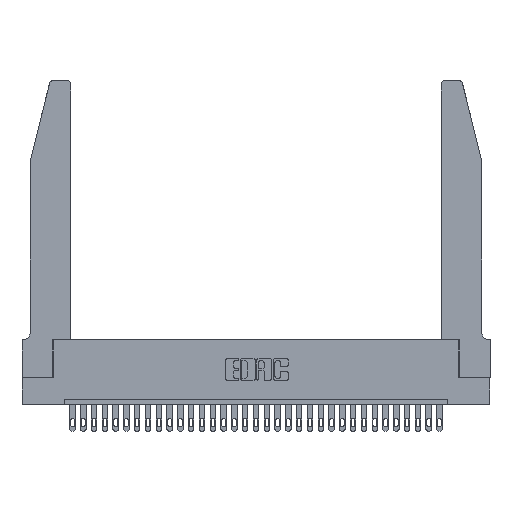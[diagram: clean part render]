
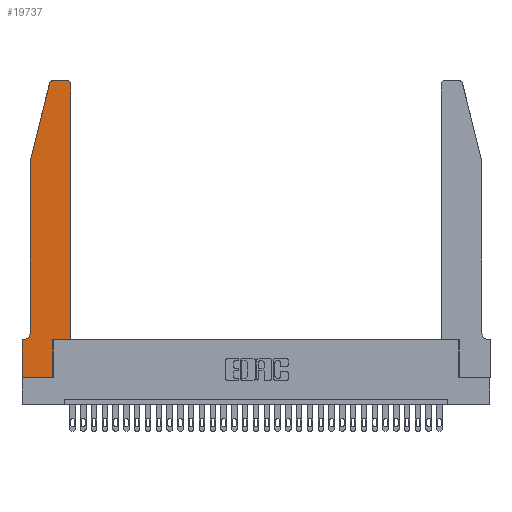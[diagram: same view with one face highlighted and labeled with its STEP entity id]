
A CAD part, top view. The second image highlights one B-rep face of the part: STEP entity #19737.
In plain terms, the highlighted planar face has unit normal (0, 0, 1).
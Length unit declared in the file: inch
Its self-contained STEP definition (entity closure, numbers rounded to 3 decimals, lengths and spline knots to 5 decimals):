
#480 = CARTESIAN_POINT ( 'NONE',  ( 0.0755, 2., 0.37 ) ) ;
#620 = CARTESIAN_POINT ( 'NONE',  ( 0.2605, 2.75, 0.37 ) ) ;
#702 = DIRECTION ( 'NONE',  ( -1., 0., 0. ) ) ;
#852 = CARTESIAN_POINT ( 'NONE',  ( 0., 0.35, 0.37 ) ) ;
#1043 = CARTESIAN_POINT ( 'NONE',  ( 0.0755, 0.42, 0.37 ) ) ;
#1354 = EDGE_CURVE ( 'NONE', #4685, #29435, #10092, .T. ) ;
#1769 = VERTEX_POINT ( 'NONE', #21962 ) ;
#2161 = EDGE_CURVE ( 'NONE', #25814, #4685, #17401, .T. ) ;
#2684 = VERTEX_POINT ( 'NONE', #5732 ) ;
#3289 = DIRECTION ( 'NONE',  ( 0., -1., 0. ) ) ;
#3474 = ORIENTED_EDGE ( 'NONE', *, *, #5643, .T. ) ;
#3964 = LINE ( 'NONE', #4809, #13573 ) ;
#4007 = CARTESIAN_POINT ( 'NONE',  ( 0.4505, 0.35, 0.37 ) ) ;
#4215 = ORIENTED_EDGE ( 'NONE', *, *, #8852, .T. ) ;
#4258 = ORIENTED_EDGE ( 'NONE', *, *, #21538, .T. ) ;
#4620 = EDGE_CURVE ( 'NONE', #2684, #25814, #16845, .T. ) ;
#4685 = VERTEX_POINT ( 'NONE', #16124 ) ;
#4809 = CARTESIAN_POINT ( 'NONE',  ( 0.4505, 0.35, 0.37 ) ) ;
#4876 = ORIENTED_EDGE ( 'NONE', *, *, #26256, .T. ) ;
#4889 = ORIENTED_EDGE ( 'NONE', *, *, #4620, .T. ) ;
#5631 = CARTESIAN_POINT ( 'NONE',  ( 0., 0.35, 0.37 ) ) ;
#5643 = EDGE_CURVE ( 'NONE', #20206, #14360, #23951, .T. ) ;
#5732 = CARTESIAN_POINT ( 'NONE',  ( 0., 0., 0.37 ) ) ;
#5796 = CARTESIAN_POINT ( 'NONE',  ( 0.0055, 0.42, 0.37 ) ) ;
#6138 = VECTOR ( 'NONE', #3289, 39.37008 ) ;
#7072 = AXIS2_PLACEMENT_3D ( 'NONE', #5796, #15475, #702 ) ;
#8675 = VERTEX_POINT ( 'NONE', #22798 ) ;
#8722 = EDGE_CURVE ( 'NONE', #1769, #20276, #18851, .T. ) ;
#8852 = EDGE_CURVE ( 'NONE', #15446, #24957, #28484, .T. ) ;
#8930 = DIRECTION ( 'NONE',  ( 0., 1., 0. ) ) ;
#9230 = DIRECTION ( 'NONE',  ( -0.239, -0.971, 0. ) ) ;
#10092 = LINE ( 'NONE', #4007, #18231 ) ;
#10106 = ORIENTED_EDGE ( 'NONE', *, *, #26439, .T. ) ;
#10431 = LINE ( 'NONE', #620, #18953 ) ;
#11023 = DIRECTION ( 'NONE',  ( 1., 0., 0. ) ) ;
#11330 = CIRCLE ( 'NONE', #7072, 0.07 ) ;
#11789 = CARTESIAN_POINT ( 'NONE',  ( 0.2865, 0., 0.37 ) ) ;
#11994 = DIRECTION ( 'NONE',  ( 1., 0., 0. ) ) ;
#12185 = ORIENTED_EDGE ( 'NONE', *, *, #26866, .T. ) ;
#12751 = FACE_OUTER_BOUND ( 'NONE', #15650, .T. ) ;
#13332 = CARTESIAN_POINT ( 'NONE',  ( 0.284, 2.72, 0.37 ) ) ;
#13545 = EDGE_CURVE ( 'NONE', #24957, #8675, #10431, .T. ) ;
#13573 = VECTOR ( 'NONE', #22075, 39.37008 ) ;
#13743 = CARTESIAN_POINT ( 'NONE',  ( 0.2865, 0.35, 0.37 ) ) ;
#14101 = VERTEX_POINT ( 'NONE', #1043 ) ;
#14218 = CARTESIAN_POINT ( 'NONE',  ( 0.4505, 2.72, 0.37 ) ) ;
#14225 = LINE ( 'NONE', #15565, #6138 ) ;
#14360 = VERTEX_POINT ( 'NONE', #480 ) ;
#15446 = VERTEX_POINT ( 'NONE', #14218 ) ;
#15475 = DIRECTION ( 'NONE',  ( 0., 0., -1. ) ) ;
#15504 = CIRCLE ( 'NONE', #27326, 0.03 ) ;
#15565 = CARTESIAN_POINT ( 'NONE',  ( 0., 0., 0.37 ) ) ;
#15650 = EDGE_LOOP ( 'NONE', ( #23477, #12185, #3474, #4876, #25760, #18470, #4258, #4889, #22389, #18075, #10106, #4215 ) ) ;
#15756 = CARTESIAN_POINT ( 'NONE',  ( 0.25487, 2.72718, 0.37 ) ) ;
#16124 = CARTESIAN_POINT ( 'NONE',  ( 0.2865, 0.35, 0.37 ) ) ;
#16845 = LINE ( 'NONE', #18393, #20302 ) ;
#16876 = DIRECTION ( 'NONE',  ( 0., 0., 1. ) ) ;
#17401 = LINE ( 'NONE', #13743, #28562 ) ;
#17899 = DIRECTION ( 'NONE',  ( -1., 0., 0. ) ) ;
#18075 = ORIENTED_EDGE ( 'NONE', *, *, #1354, .T. ) ;
#18154 = AXIS2_PLACEMENT_3D ( 'NONE', #852, #23378, #25742 ) ;
#18231 = VECTOR ( 'NONE', #19000, 39.37008 ) ;
#18257 = DIRECTION ( 'NONE',  ( 0., 0., 1. ) ) ;
#18393 = CARTESIAN_POINT ( 'NONE',  ( 0., 0., 0.37 ) ) ;
#18470 = ORIENTED_EDGE ( 'NONE', *, *, #8722, .T. ) ;
#18851 = LINE ( 'NONE', #20424, #28876 ) ;
#18953 = VECTOR ( 'NONE', #17899, 39.37008 ) ;
#19000 = DIRECTION ( 'NONE',  ( 1., 0., 0. ) ) ;
#19737 = ADVANCED_FACE ( 'NONE', ( #12751 ), #27813, .T. ) ;
#20206 = VERTEX_POINT ( 'NONE', #15756 ) ;
#20276 = VERTEX_POINT ( 'NONE', #5631 ) ;
#20302 = VECTOR ( 'NONE', #11023, 39.37008 ) ;
#20424 = CARTESIAN_POINT ( 'NONE',  ( 0.0755, 0.35, 0.37 ) ) ;
#21538 = EDGE_CURVE ( 'NONE', #20276, #2684, #14225, .T. ) ;
#21962 = CARTESIAN_POINT ( 'NONE',  ( 0.0055, 0.35, 0.37 ) ) ;
#22075 = DIRECTION ( 'NONE',  ( 0., 1., 0. ) ) ;
#22389 = ORIENTED_EDGE ( 'NONE', *, *, #2161, .T. ) ;
#22798 = CARTESIAN_POINT ( 'NONE',  ( 0.284, 2.75, 0.37 ) ) ;
#23213 = DIRECTION ( 'NONE',  ( -1., 0., 0. ) ) ;
#23378 = DIRECTION ( 'NONE',  ( 0., 0., 1. ) ) ;
#23477 = ORIENTED_EDGE ( 'NONE', *, *, #13545, .T. ) ;
#23653 = DIRECTION ( 'NONE',  ( 0., -1., 0. ) ) ;
#23655 = EDGE_CURVE ( 'NONE', #14101, #1769, #11330, .T. ) ;
#23951 = LINE ( 'NONE', #31430, #26265 ) ;
#24794 = VECTOR ( 'NONE', #23653, 39.37008 ) ;
#24957 = VERTEX_POINT ( 'NONE', #28556 ) ;
#25171 = LINE ( 'NONE', #30869, #24794 ) ;
#25742 = DIRECTION ( 'NONE',  ( 1., 0., 0. ) ) ;
#25760 = ORIENTED_EDGE ( 'NONE', *, *, #23655, .T. ) ;
#25814 = VERTEX_POINT ( 'NONE', #11789 ) ;
#26256 = EDGE_CURVE ( 'NONE', #14360, #14101, #25171, .T. ) ;
#26265 = VECTOR ( 'NONE', #9230, 39.37008 ) ;
#26439 = EDGE_CURVE ( 'NONE', #29435, #15446, #3964, .T. ) ;
#26449 = CARTESIAN_POINT ( 'NONE',  ( 0.4205, 2.72, 0.37 ) ) ;
#26866 = EDGE_CURVE ( 'NONE', #8675, #20206, #15504, .T. ) ;
#27326 = AXIS2_PLACEMENT_3D ( 'NONE', #13332, #18257, #30616 ) ;
#27813 = PLANE ( 'NONE',  #18154 ) ;
#28198 = CARTESIAN_POINT ( 'NONE',  ( 0.4505, 0.35, 0.37 ) ) ;
#28484 = CIRCLE ( 'NONE', #28674, 0.03 ) ;
#28556 = CARTESIAN_POINT ( 'NONE',  ( 0.4205, 2.75, 0.37 ) ) ;
#28562 = VECTOR ( 'NONE', #8930, 39.37008 ) ;
#28674 = AXIS2_PLACEMENT_3D ( 'NONE', #26449, #16876, #11994 ) ;
#28876 = VECTOR ( 'NONE', #23213, 39.37008 ) ;
#29435 = VERTEX_POINT ( 'NONE', #28198 ) ;
#30616 = DIRECTION ( 'NONE',  ( 1., 0., 0. ) ) ;
#30869 = CARTESIAN_POINT ( 'NONE',  ( 0.0755, 2., 0.37 ) ) ;
#31430 = CARTESIAN_POINT ( 'NONE',  ( 0.0755, 2., 0.37 ) ) ;
